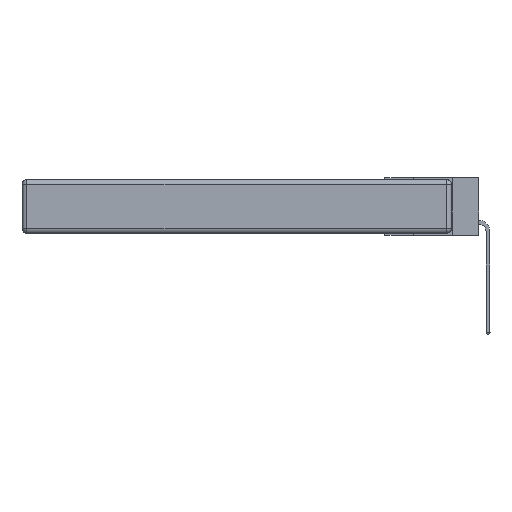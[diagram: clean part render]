
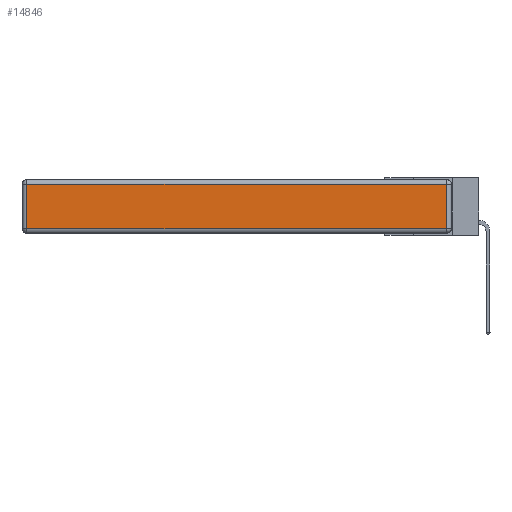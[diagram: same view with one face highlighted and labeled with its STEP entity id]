
A CAD part, left-side view. The second image highlights one B-rep face of the part: STEP entity #14846.
In plain terms, the highlighted planar face has unit normal (-1, 0, 0).
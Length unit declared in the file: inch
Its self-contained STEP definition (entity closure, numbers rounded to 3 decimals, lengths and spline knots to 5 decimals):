
#920 = PLANE ( 'NONE',  #22753 ) ;
#2024 = DIRECTION ( 'NONE',  ( 0., -1., 0. ) ) ;
#2130 = VECTOR ( 'NONE', #3077, 39.37008 ) ;
#2615 = FACE_OUTER_BOUND ( 'NONE', #7958, .T. ) ;
#2717 = ORIENTED_EDGE ( 'NONE', *, *, #20519, .T. ) ;
#2998 = VECTOR ( 'NONE', #18388, 39.37008 ) ;
#3077 = DIRECTION ( 'NONE',  ( 0., 0., -1. ) ) ;
#3192 = ORIENTED_EDGE ( 'NONE', *, *, #9160, .T. ) ;
#6227 = VECTOR ( 'NONE', #2024, 39.37008 ) ;
#6558 = VERTEX_POINT ( 'NONE', #25073 ) ;
#7958 = EDGE_LOOP ( 'NONE', ( #3192, #24085, #25577, #2717 ) ) ;
#9160 = EDGE_CURVE ( 'NONE', #17120, #6558, #18798, .T. ) ;
#10158 = DIRECTION ( 'NONE',  ( 0., 0., 1. ) ) ;
#11170 = VECTOR ( 'NONE', #10158, 39.37008 ) ;
#12401 = EDGE_CURVE ( 'NONE', #18983, #20118, #14106, .T. ) ;
#14030 = EDGE_CURVE ( 'NONE', #6558, #18983, #20423, .T. ) ;
#14106 = LINE ( 'NONE', #18292, #2998 ) ;
#14846 = ADVANCED_FACE ( 'NONE', ( #2615 ), #920, .T. ) ;
#16192 = CARTESIAN_POINT ( 'NONE',  ( 0., 0., -0.313 ) ) ;
#17052 = DIRECTION ( 'NONE',  ( 0., 0., 1. ) ) ;
#17120 = VERTEX_POINT ( 'NONE', #19811 ) ;
#18292 = CARTESIAN_POINT ( 'NONE',  ( 0., 2.75, -0.03 ) ) ;
#18388 = DIRECTION ( 'NONE',  ( 0., 1., 0. ) ) ;
#18798 = LINE ( 'NONE', #16192, #6227 ) ;
#18983 = VERTEX_POINT ( 'NONE', #30484 ) ;
#19391 = CARTESIAN_POINT ( 'NONE',  ( 0., 0.03, -0.343 ) ) ;
#19811 = CARTESIAN_POINT ( 'NONE',  ( 0., 2.72, -0.313 ) ) ;
#20118 = VERTEX_POINT ( 'NONE', #30179 ) ;
#20423 = LINE ( 'NONE', #19391, #11170 ) ;
#20519 = EDGE_CURVE ( 'NONE', #20118, #17120, #29761, .T. ) ;
#22753 = AXIS2_PLACEMENT_3D ( 'NONE', #26630, #26537, #17052 ) ;
#24085 = ORIENTED_EDGE ( 'NONE', *, *, #14030, .T. ) ;
#25073 = CARTESIAN_POINT ( 'NONE',  ( 0., 0.03, -0.313 ) ) ;
#25577 = ORIENTED_EDGE ( 'NONE', *, *, #12401, .T. ) ;
#26537 = DIRECTION ( 'NONE',  ( -1., 0., 0. ) ) ;
#26630 = CARTESIAN_POINT ( 'NONE',  ( 0., 0., -0.343 ) ) ;
#26934 = CARTESIAN_POINT ( 'NONE',  ( 0., 2.72, -0.343 ) ) ;
#29761 = LINE ( 'NONE', #26934, #2130 ) ;
#30179 = CARTESIAN_POINT ( 'NONE',  ( 0., 2.72, -0.03 ) ) ;
#30484 = CARTESIAN_POINT ( 'NONE',  ( 0., 0.03, -0.03 ) ) ;
